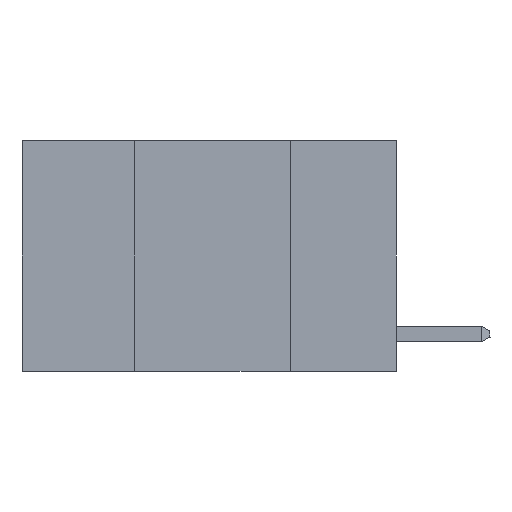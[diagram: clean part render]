
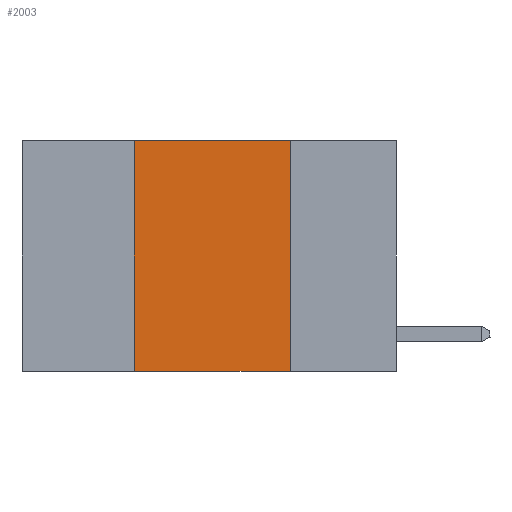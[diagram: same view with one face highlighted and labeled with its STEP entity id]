
A CAD part, left-side view. The second image highlights one B-rep face of the part: STEP entity #2003.
In plain terms, the highlighted planar face has unit normal (-1, 0, 0).
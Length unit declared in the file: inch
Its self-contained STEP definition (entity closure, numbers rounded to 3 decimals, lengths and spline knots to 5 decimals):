
#203 = CARTESIAN_POINT ( 'NONE',  ( 0., 0.42, 0. ) ) ;
#445 = CARTESIAN_POINT ( 'NONE',  ( 0., 0.17, 0. ) ) ;
#588 = VERTEX_POINT ( 'NONE', #6258 ) ;
#634 = VECTOR ( 'NONE', #7914, 39.37008 ) ;
#1032 = CARTESIAN_POINT ( 'NONE',  ( 0., 0.6, 0. ) ) ;
#1441 = VERTEX_POINT ( 'NONE', #3178 ) ;
#1829 = AXIS2_PLACEMENT_3D ( 'NONE', #1032, #6701, #11499 ) ;
#1877 = EDGE_CURVE ( 'NONE', #1441, #2098, #10728, .T. ) ;
#2003 = ADVANCED_FACE ( 'NONE', ( #4355 ), #3451, .F. ) ;
#2098 = VERTEX_POINT ( 'NONE', #445 ) ;
#2130 = LINE ( 'NONE', #7710, #6551 ) ;
#3178 = CARTESIAN_POINT ( 'NONE',  ( 0., 0.42, 0. ) ) ;
#3451 = PLANE ( 'NONE',  #1829 ) ;
#4137 = ORIENTED_EDGE ( 'NONE', *, *, #10912, .T. ) ;
#4211 = DIRECTION ( 'NONE',  ( 0., 0., 1. ) ) ;
#4311 = DIRECTION ( 'NONE',  ( 0., -1., 0. ) ) ;
#4355 = FACE_OUTER_BOUND ( 'NONE', #10622, .T. ) ;
#4364 = CARTESIAN_POINT ( 'NONE',  ( 0., 0.6, 0. ) ) ;
#4677 = ORIENTED_EDGE ( 'NONE', *, *, #11336, .F. ) ;
#4995 = DIRECTION ( 'NONE',  ( 0., 0., -1. ) ) ;
#5930 = CARTESIAN_POINT ( 'NONE',  ( 0., 0.6, -0.37 ) ) ;
#6258 = CARTESIAN_POINT ( 'NONE',  ( 0., 0.17, -0.37 ) ) ;
#6551 = VECTOR ( 'NONE', #4995, 39.37008 ) ;
#6701 = DIRECTION ( 'NONE',  ( 1., 0., 0. ) ) ;
#6834 = ORIENTED_EDGE ( 'NONE', *, *, #8915, .F. ) ;
#7103 = VECTOR ( 'NONE', #4311, 39.37008 ) ;
#7710 = CARTESIAN_POINT ( 'NONE',  ( 0., 0.17, 0. ) ) ;
#7914 = DIRECTION ( 'NONE',  ( 0., -1., 0. ) ) ;
#8915 = EDGE_CURVE ( 'NONE', #9675, #1441, #11559, .T. ) ;
#9494 = LINE ( 'NONE', #5930, #634 ) ;
#9675 = VERTEX_POINT ( 'NONE', #11355 ) ;
#10310 = ORIENTED_EDGE ( 'NONE', *, *, #1877, .F. ) ;
#10622 = EDGE_LOOP ( 'NONE', ( #4677, #10310, #6834, #4137 ) ) ;
#10728 = LINE ( 'NONE', #4364, #7103 ) ;
#10912 = EDGE_CURVE ( 'NONE', #9675, #588, #9494, .T. ) ;
#11336 = EDGE_CURVE ( 'NONE', #2098, #588, #2130, .T. ) ;
#11355 = CARTESIAN_POINT ( 'NONE',  ( 0., 0.42, -0.37 ) ) ;
#11499 = DIRECTION ( 'NONE',  ( 0., 0., -1. ) ) ;
#11559 = LINE ( 'NONE', #203, #11715 ) ;
#11715 = VECTOR ( 'NONE', #4211, 39.37008 ) ;
